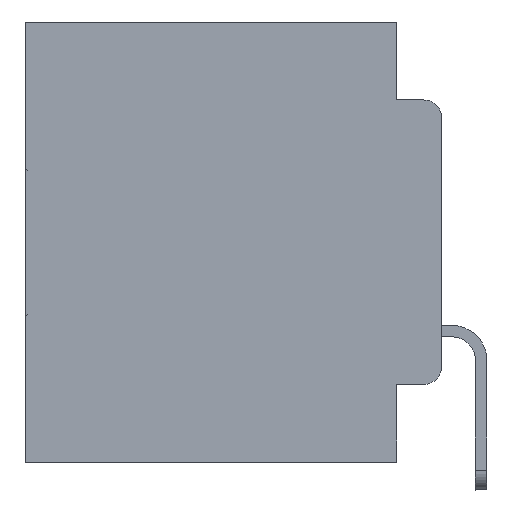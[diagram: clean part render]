
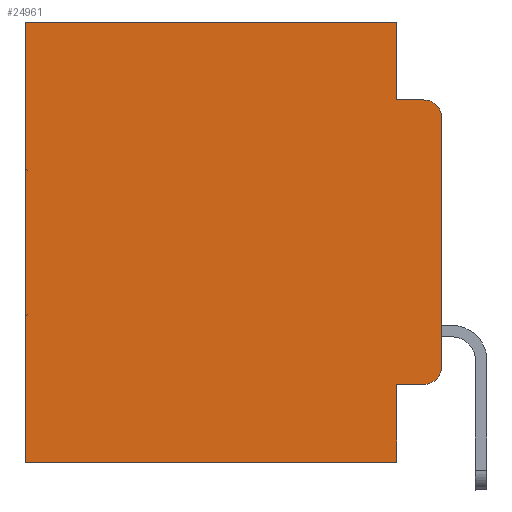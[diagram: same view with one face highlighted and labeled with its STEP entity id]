
A CAD part, left-side view. The second image highlights one B-rep face of the part: STEP entity #24961.
In plain terms, the highlighted planar face has unit normal (-1, 0, 0).
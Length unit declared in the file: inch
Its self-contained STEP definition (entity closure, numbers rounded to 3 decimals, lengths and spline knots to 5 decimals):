
#325 = EDGE_LOOP ( 'NONE', ( #21815, #18046, #6527, #12228, #9892, #13992, #26977, #2519, #30806, #17396 ) ) ;
#598 = DIRECTION ( 'NONE',  ( 0., -1., 0. ) ) ;
#831 = VECTOR ( 'NONE', #598, 39.37008 ) ;
#1404 = DIRECTION ( 'NONE',  ( 1., 0., 0. ) ) ;
#1768 = DIRECTION ( 'NONE',  ( 0., 1., 0. ) ) ;
#1984 = CARTESIAN_POINT ( 'NONE',  ( 0.298, 0.051, -0.0885 ) ) ;
#2038 = LINE ( 'NONE', #2347, #20502 ) ;
#2347 = CARTESIAN_POINT ( 'NONE',  ( 0.298, 0.051, 0. ) ) ;
#2353 = EDGE_CURVE ( 'NONE', #15008, #20280, #2038, .T. ) ;
#2519 = ORIENTED_EDGE ( 'NONE', *, *, #10627, .F. ) ;
#2753 = AXIS2_PLACEMENT_3D ( 'NONE', #28761, #1404, #30670 ) ;
#2841 = CARTESIAN_POINT ( 'NONE',  ( 0.298, 0.02, -0.1085 ) ) ;
#3217 = EDGE_CURVE ( 'NONE', #20280, #16201, #9460, .T. ) ;
#3240 = VERTEX_POINT ( 'NONE', #26139 ) ;
#3838 = LINE ( 'NONE', #13222, #23109 ) ;
#4069 = VECTOR ( 'NONE', #13218, 39.37008 ) ;
#4114 = PLANE ( 'NONE',  #2753 ) ;
#4210 = VERTEX_POINT ( 'NONE', #26962 ) ;
#4596 = VERTEX_POINT ( 'NONE', #5463 ) ;
#5463 = CARTESIAN_POINT ( 'NONE',  ( 0.298, 0.473, 0. ) ) ;
#5725 = VERTEX_POINT ( 'NONE', #8876 ) ;
#6473 = CARTESIAN_POINT ( 'NONE',  ( 0.298, 0.02, -0.3915 ) ) ;
#6527 = ORIENTED_EDGE ( 'NONE', *, *, #3217, .F. ) ;
#8355 = VECTOR ( 'NONE', #12715, 39.37008 ) ;
#8482 = CARTESIAN_POINT ( 'NONE',  ( 0.298, 0.051, 0. ) ) ;
#8876 = CARTESIAN_POINT ( 'NONE',  ( 0.298, 0.02, -0.4115 ) ) ;
#9133 = EDGE_CURVE ( 'NONE', #5725, #23719, #19887, .T. ) ;
#9460 = LINE ( 'NONE', #13906, #17323 ) ;
#9672 = CARTESIAN_POINT ( 'NONE',  ( 0.298, 0., 0. ) ) ;
#9703 = LINE ( 'NONE', #19381, #831 ) ;
#9892 = ORIENTED_EDGE ( 'NONE', *, *, #16245, .T. ) ;
#10264 = AXIS2_PLACEMENT_3D ( 'NONE', #2841, #16845, #19696 ) ;
#10603 = DIRECTION ( 'NONE',  ( -1., 0., 0. ) ) ;
#10627 = EDGE_CURVE ( 'NONE', #4210, #12816, #27863, .T. ) ;
#10743 = CARTESIAN_POINT ( 'NONE',  ( 0.298, 0.051, 0. ) ) ;
#11259 = CARTESIAN_POINT ( 'NONE',  ( 0.298, 0., -0.3915 ) ) ;
#12228 = ORIENTED_EDGE ( 'NONE', *, *, #2353, .F. ) ;
#12715 = DIRECTION ( 'NONE',  ( 0., 1., 0. ) ) ;
#12816 = VERTEX_POINT ( 'NONE', #13305 ) ;
#13218 = DIRECTION ( 'NONE',  ( 0., 0., -1. ) ) ;
#13222 = CARTESIAN_POINT ( 'NONE',  ( 0.298, 0., -0.5 ) ) ;
#13305 = CARTESIAN_POINT ( 'NONE',  ( 0.298, 0.051, -0.5 ) ) ;
#13833 = EDGE_CURVE ( 'NONE', #3240, #16201, #18387, .T. ) ;
#13906 = CARTESIAN_POINT ( 'NONE',  ( 0.298, 0.051, -0.0885 ) ) ;
#13992 = ORIENTED_EDGE ( 'NONE', *, *, #24829, .T. ) ;
#15008 = VERTEX_POINT ( 'NONE', #10743 ) ;
#16201 = VERTEX_POINT ( 'NONE', #31328 ) ;
#16245 = EDGE_CURVE ( 'NONE', #15008, #4596, #17655, .T. ) ;
#16298 = DIRECTION ( 'NONE',  ( 0., -1., 0. ) ) ;
#16845 = DIRECTION ( 'NONE',  ( -1., 0., 0. ) ) ;
#16990 = DIRECTION ( 'NONE',  ( 0., 0., -1. ) ) ;
#17323 = VECTOR ( 'NONE', #16298, 39.37008 ) ;
#17396 = ORIENTED_EDGE ( 'NONE', *, *, #9133, .T. ) ;
#17655 = LINE ( 'NONE', #29728, #8355 ) ;
#17958 = LINE ( 'NONE', #22883, #22034 ) ;
#18046 = ORIENTED_EDGE ( 'NONE', *, *, #13833, .T. ) ;
#18387 = CIRCLE ( 'NONE', #10264, 0.02 ) ;
#19381 = CARTESIAN_POINT ( 'NONE',  ( 0.298, 0.051, -0.4115 ) ) ;
#19554 = EDGE_CURVE ( 'NONE', #4210, #5725, #9703, .T. ) ;
#19696 = DIRECTION ( 'NONE',  ( 0., 0., -1. ) ) ;
#19887 = CIRCLE ( 'NONE', #23942, 0.02 ) ;
#19892 = VERTEX_POINT ( 'NONE', #25875 ) ;
#20280 = VERTEX_POINT ( 'NONE', #1984 ) ;
#20502 = VECTOR ( 'NONE', #16990, 39.37008 ) ;
#21434 = FACE_OUTER_BOUND ( 'NONE', #325, .T. ) ;
#21815 = ORIENTED_EDGE ( 'NONE', *, *, #22531, .F. ) ;
#21880 = LINE ( 'NONE', #9672, #24512 ) ;
#22034 = VECTOR ( 'NONE', #22728, 39.37008 ) ;
#22531 = EDGE_CURVE ( 'NONE', #3240, #23719, #21880, .T. ) ;
#22728 = DIRECTION ( 'NONE',  ( 0., 0., -1. ) ) ;
#22883 = CARTESIAN_POINT ( 'NONE',  ( 0.298, 0.473, 0. ) ) ;
#23109 = VECTOR ( 'NONE', #1768, 39.37008 ) ;
#23320 = DIRECTION ( 'NONE',  ( 0., 0., -1. ) ) ;
#23719 = VERTEX_POINT ( 'NONE', #11259 ) ;
#23942 = AXIS2_PLACEMENT_3D ( 'NONE', #6473, #10603, #23320 ) ;
#24512 = VECTOR ( 'NONE', #31441, 39.37008 ) ;
#24829 = EDGE_CURVE ( 'NONE', #4596, #19892, #17958, .T. ) ;
#24961 = ADVANCED_FACE ( 'NONE', ( #21434 ), #4114, .F. ) ;
#25875 = CARTESIAN_POINT ( 'NONE',  ( 0.298, 0.473, -0.5 ) ) ;
#26139 = CARTESIAN_POINT ( 'NONE',  ( 0.298, 0., -0.1085 ) ) ;
#26150 = EDGE_CURVE ( 'NONE', #12816, #19892, #3838, .T. ) ;
#26962 = CARTESIAN_POINT ( 'NONE',  ( 0.298, 0.051, -0.4115 ) ) ;
#26977 = ORIENTED_EDGE ( 'NONE', *, *, #26150, .F. ) ;
#27863 = LINE ( 'NONE', #8482, #4069 ) ;
#28761 = CARTESIAN_POINT ( 'NONE',  ( 0.298, 0., 0. ) ) ;
#29728 = CARTESIAN_POINT ( 'NONE',  ( 0.298, 0., 0. ) ) ;
#30670 = DIRECTION ( 'NONE',  ( 0., 0., -1. ) ) ;
#30806 = ORIENTED_EDGE ( 'NONE', *, *, #19554, .T. ) ;
#31328 = CARTESIAN_POINT ( 'NONE',  ( 0.298, 0.02, -0.0885 ) ) ;
#31441 = DIRECTION ( 'NONE',  ( 0., 0., -1. ) ) ;
